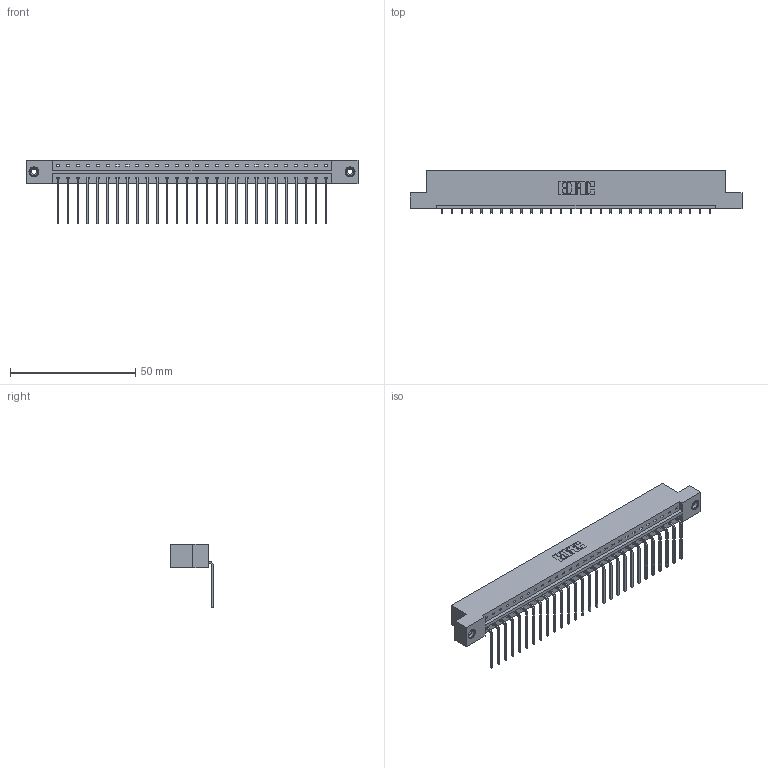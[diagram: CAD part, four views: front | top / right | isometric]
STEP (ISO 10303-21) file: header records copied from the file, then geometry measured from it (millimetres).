
FILE_DESCRIPTION (( 'STEP AP203' ), '1' );
FILE_NAME ('833-028-559-108.STEP', '2020-06-02T09:59:40', ( '' ), ( '' ), 'SwSTEP 2.0', 'SolidWorks 2020', '' );
FILE_SCHEMA (( 'CONFIG_CONTROL_DESIGN' ));
Length unit declared in the file: inch
Products named in the file (4): 833 Part_Flush - .156 Dia - TI; 833-028-559-108; 345-250-001_345-250-003-102; 345-292-001_558 559 Tail - 1
Assembly tree (31 placements, depth 2):
  833-028-559-108
    833 Part_Flush - .156 Dia - TI
    345-292-001_558 559 Tail - 1  x28
    345-250-001_345-250-003-102  x2
Bounding box: 132.49 x 17.09 x 25.53 mm (x, y, z)
Volume: 13298.2 mm3; surface area: 14894.7 mm2
Topology: 31 solids, 31 shells, 1854 faces, 5543 edges, 3650 vertices
Faces by surface type: plane 1334, cylinder 504, cone 12, torus 4
Entity records: 20198 total; most frequent: CARTESIAN_POINT 3469, ORIENTED_EDGE 3426, DIRECTION 2987, EDGE_CURVE 1713, LINE 1565, VECTOR 1565, VERTEX_POINT 1136, AXIS2_PLACEMENT_3D 711
